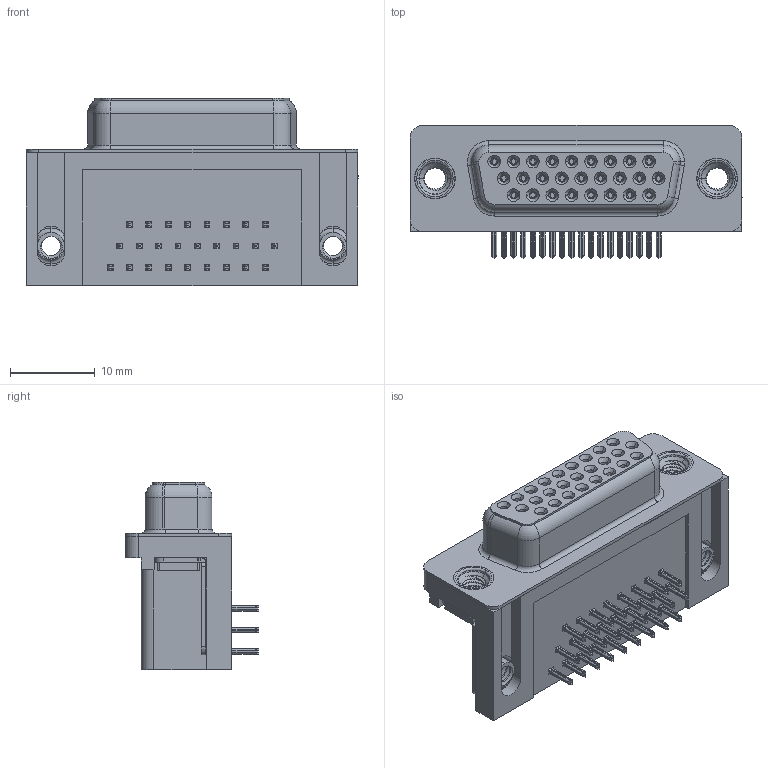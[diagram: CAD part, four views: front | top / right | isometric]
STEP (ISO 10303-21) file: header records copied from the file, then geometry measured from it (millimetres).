
FILE_DESCRIPTION (( 'STEP AP203' ), '1' );
FILE_NAME ('634-026-363-555.STEP', '2018-11-09T23:49:48', ( '' ), ( '' ), 'SwSTEP 2.0', 'SolidWorks 2016', '' );
FILE_SCHEMA (( 'CONFIG_CONTROL_DESIGN' ));
Length unit declared in the file: millimetre
Products named in the file (8): 634 Shell_26 Socket; Contact Bottom; Contact Middle; 634 Housing_26 Socket; Contact Top; 4-40 Threaded Board Mount; 634-026-363-555; M3 Threaded Rivet
Assembly tree (32 placements, depth 2):
  634-026-363-555
    634 Housing_26 Socket
    634 Shell_26 Socket
    Contact Bottom  x8
    Contact Middle  x9
    Contact Top  x9
    4-40 Threaded Board Mount  x2
    M3 Threaded Rivet  x2
Bounding box: 39.22 x 15.73 x 22.1 mm (x, y, z)
Volume: 6372.3 mm3; surface area: 9163 mm2
Topology: 32 solids, 32 shells, 4011 faces, 10548 edges, 6628 vertices
Faces by surface type: plane 1771, cylinder 954, bspline 916, cone 320, torus 50
Entity records: 38243 total; most frequent: CARTESIAN_POINT 13460, ORIENTED_EDGE 5044, DIRECTION 4432, EDGE_CURVE 2522, VERTEX_POINT 1607, LINE 1582, VECTOR 1582, AXIS2_PLACEMENT_3D 1425
